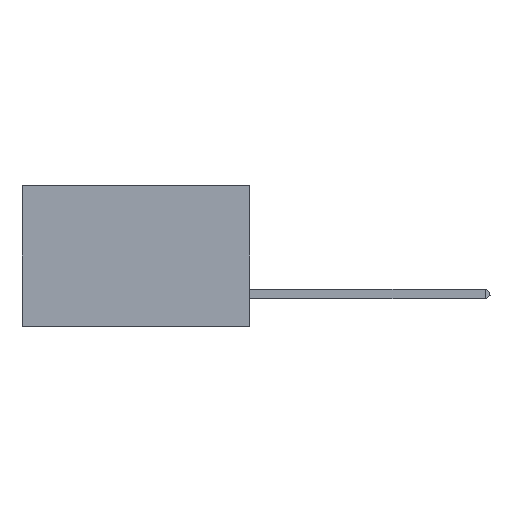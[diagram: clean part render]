
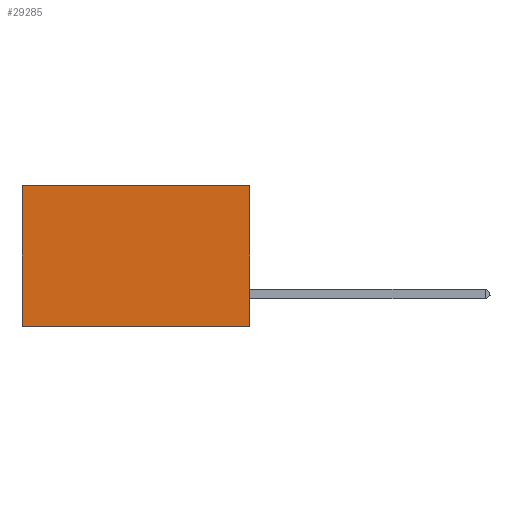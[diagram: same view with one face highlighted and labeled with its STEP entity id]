
A CAD part, left-side view. The second image highlights one B-rep face of the part: STEP entity #29285.
In plain terms, the highlighted planar face has unit normal (-1, 0, 0).
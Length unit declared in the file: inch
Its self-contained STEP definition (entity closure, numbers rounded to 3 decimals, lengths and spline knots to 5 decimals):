
#1283 = EDGE_CURVE ( 'NONE', #10510, #24798, #32275, .T. ) ;
#1365 = DIRECTION ( 'NONE',  ( 0., 0., -1. ) ) ;
#2203 = EDGE_CURVE ( 'NONE', #8189, #24798, #16058, .T. ) ;
#2465 = CARTESIAN_POINT ( 'NONE',  ( 0.2875, 0., -0.37 ) ) ;
#3000 = VECTOR ( 'NONE', #1365, 39.37008 ) ;
#4274 = ORIENTED_EDGE ( 'NONE', *, *, #30462, .F. ) ;
#4569 = CARTESIAN_POINT ( 'NONE',  ( 0.2875, 0., -0.37 ) ) ;
#6434 = EDGE_CURVE ( 'NONE', #19387, #10510, #40954, .T. ) ;
#6976 = PLANE ( 'NONE',  #38134 ) ;
#7480 = ORIENTED_EDGE ( 'NONE', *, *, #6434, .T. ) ;
#7584 = VECTOR ( 'NONE', #33172, 39.37008 ) ;
#8189 = VERTEX_POINT ( 'NONE', #2465 ) ;
#10350 = DIRECTION ( 'NONE',  ( 1., 0., 0. ) ) ;
#10510 = VERTEX_POINT ( 'NONE', #26177 ) ;
#11644 = DIRECTION ( 'NONE',  ( 0., 1., 0. ) ) ;
#11792 = ORIENTED_EDGE ( 'NONE', *, *, #1283, .T. ) ;
#12005 = CARTESIAN_POINT ( 'NONE',  ( 0.2875, 0., 0. ) ) ;
#15657 = VECTOR ( 'NONE', #34587, 39.37008 ) ;
#16058 = LINE ( 'NONE', #4569, #34433 ) ;
#18115 = CARTESIAN_POINT ( 'NONE',  ( 0.2875, 0., 0. ) ) ;
#19387 = VERTEX_POINT ( 'NONE', #12005 ) ;
#19678 = CARTESIAN_POINT ( 'NONE',  ( 0.2875, 0., 0. ) ) ;
#24798 = VERTEX_POINT ( 'NONE', #36331 ) ;
#26177 = CARTESIAN_POINT ( 'NONE',  ( 0.2875, 0.6, 0. ) ) ;
#29285 = ADVANCED_FACE ( 'NONE', ( #40588 ), #6976, .F. ) ;
#29829 = EDGE_LOOP ( 'NONE', ( #11792, #41017, #4274, #7480 ) ) ;
#30462 = EDGE_CURVE ( 'NONE', #19387, #8189, #30540, .T. ) ;
#30540 = LINE ( 'NONE', #18115, #7584 ) ;
#32275 = LINE ( 'NONE', #45309, #3000 ) ;
#33172 = DIRECTION ( 'NONE',  ( 0., 0., -1. ) ) ;
#34433 = VECTOR ( 'NONE', #11644, 39.37008 ) ;
#34587 = DIRECTION ( 'NONE',  ( 0., 1., 0. ) ) ;
#36331 = CARTESIAN_POINT ( 'NONE',  ( 0.2875, 0.6, -0.37 ) ) ;
#38134 = AXIS2_PLACEMENT_3D ( 'NONE', #46922, #10350, #47400 ) ;
#40588 = FACE_OUTER_BOUND ( 'NONE', #29829, .T. ) ;
#40954 = LINE ( 'NONE', #19678, #15657 ) ;
#41017 = ORIENTED_EDGE ( 'NONE', *, *, #2203, .F. ) ;
#45309 = CARTESIAN_POINT ( 'NONE',  ( 0.2875, 0.6, 0. ) ) ;
#46922 = CARTESIAN_POINT ( 'NONE',  ( 0.2875, 0., 0. ) ) ;
#47400 = DIRECTION ( 'NONE',  ( 0., 0., -1. ) ) ;
